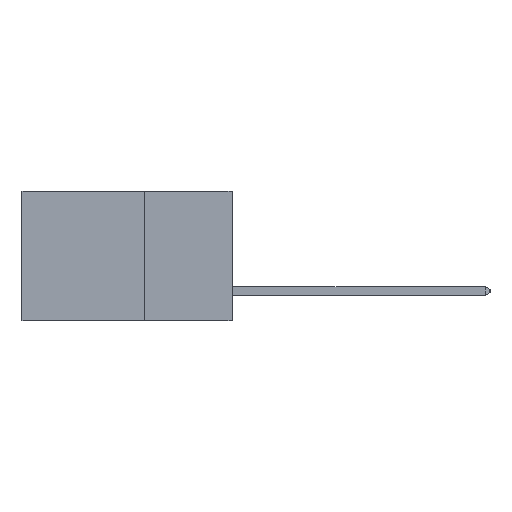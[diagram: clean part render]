
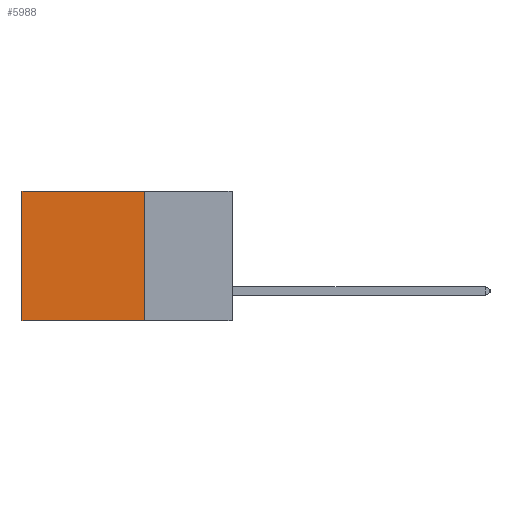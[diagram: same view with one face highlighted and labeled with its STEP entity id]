
A CAD part, left-side view. The second image highlights one B-rep face of the part: STEP entity #5988.
In plain terms, the highlighted planar face has unit normal (-1, 0, 0).
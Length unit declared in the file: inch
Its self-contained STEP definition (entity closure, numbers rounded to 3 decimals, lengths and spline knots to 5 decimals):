
#1230 = CARTESIAN_POINT ( 'NONE',  ( 0.2875, 0.25, 0. ) ) ;
#1961 = DIRECTION ( 'NONE',  ( 0., 0., -1. ) ) ;
#2511 = VECTOR ( 'NONE', #29660, 39.37008 ) ;
#2609 = EDGE_CURVE ( 'NONE', #3541, #18223, #33926, .T. ) ;
#3122 = CARTESIAN_POINT ( 'NONE',  ( 0.2875, 0.25, -0.37 ) ) ;
#3541 = VERTEX_POINT ( 'NONE', #31096 ) ;
#4602 = CARTESIAN_POINT ( 'NONE',  ( 0.2875, 0.6, 0. ) ) ;
#5988 = ADVANCED_FACE ( 'NONE', ( #36621 ), #23429, .F. ) ;
#6037 = ORIENTED_EDGE ( 'NONE', *, *, #36396, .T. ) ;
#7239 = ORIENTED_EDGE ( 'NONE', *, *, #2609, .F. ) ;
#8479 = DIRECTION ( 'NONE',  ( 0., 0., -1. ) ) ;
#9502 = EDGE_LOOP ( 'NONE', ( #6037, #7239, #14299, #25267 ) ) ;
#9679 = LINE ( 'NONE', #27538, #16155 ) ;
#12932 = VECTOR ( 'NONE', #28211, 39.37008 ) ;
#14299 = ORIENTED_EDGE ( 'NONE', *, *, #28949, .F. ) ;
#15241 = VERTEX_POINT ( 'NONE', #38416 ) ;
#16155 = VECTOR ( 'NONE', #8479, 39.37008 ) ;
#17522 = EDGE_CURVE ( 'NONE', #34329, #15241, #25839, .T. ) ;
#18223 = VERTEX_POINT ( 'NONE', #38179 ) ;
#18756 = VECTOR ( 'NONE', #1961, 39.37008 ) ;
#20508 = DIRECTION ( 'NONE',  ( 1., 0., 0. ) ) ;
#23429 = PLANE ( 'NONE',  #27059 ) ;
#23732 = LINE ( 'NONE', #4602, #18756 ) ;
#25267 = ORIENTED_EDGE ( 'NONE', *, *, #17522, .T. ) ;
#25839 = LINE ( 'NONE', #34923, #12932 ) ;
#26754 = DIRECTION ( 'NONE',  ( 0., 0., -1. ) ) ;
#27059 = AXIS2_PLACEMENT_3D ( 'NONE', #39076, #20508, #26754 ) ;
#27538 = CARTESIAN_POINT ( 'NONE',  ( 0.2875, 0.25, 0. ) ) ;
#28211 = DIRECTION ( 'NONE',  ( 0., 1., 0. ) ) ;
#28949 = EDGE_CURVE ( 'NONE', #34329, #3541, #9679, .T. ) ;
#29660 = DIRECTION ( 'NONE',  ( 0., 1., 0. ) ) ;
#31096 = CARTESIAN_POINT ( 'NONE',  ( 0.2875, 0.25, -0.37 ) ) ;
#33926 = LINE ( 'NONE', #3122, #2511 ) ;
#34329 = VERTEX_POINT ( 'NONE', #1230 ) ;
#34923 = CARTESIAN_POINT ( 'NONE',  ( 0.2875, 0.25, 0. ) ) ;
#36396 = EDGE_CURVE ( 'NONE', #15241, #18223, #23732, .T. ) ;
#36621 = FACE_OUTER_BOUND ( 'NONE', #9502, .T. ) ;
#38179 = CARTESIAN_POINT ( 'NONE',  ( 0.2875, 0.6, -0.37 ) ) ;
#38416 = CARTESIAN_POINT ( 'NONE',  ( 0.2875, 0.6, 0. ) ) ;
#39076 = CARTESIAN_POINT ( 'NONE',  ( 0.2875, 0.25, 0. ) ) ;
